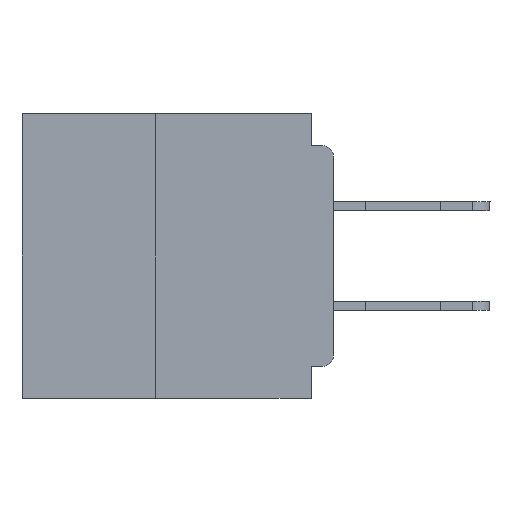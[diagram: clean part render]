
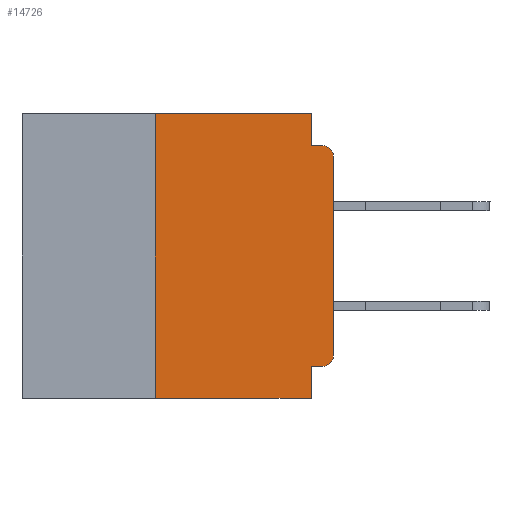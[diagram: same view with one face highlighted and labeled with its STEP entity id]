
A CAD part, left-side view. The second image highlights one B-rep face of the part: STEP entity #14726.
In plain terms, the highlighted planar face has unit normal (-1, 0, 0).
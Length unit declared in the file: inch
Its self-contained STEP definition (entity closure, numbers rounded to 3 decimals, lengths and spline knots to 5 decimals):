
#247 = VECTOR ( 'NONE', #10083, 39.37008 ) ;
#314 = FACE_OUTER_BOUND ( 'NONE', #32976, .T. ) ;
#708 = LINE ( 'NONE', #953, #49015 ) ;
#953 = CARTESIAN_POINT ( 'NONE',  ( 0., 0., -0.045 ) ) ;
#1011 = CARTESIAN_POINT ( 'NONE',  ( 0., 0.031, -0.4 ) ) ;
#1020 = LINE ( 'NONE', #16061, #47851 ) ;
#1048 = ORIENTED_EDGE ( 'NONE', *, *, #45016, .F. ) ;
#1842 = CARTESIAN_POINT ( 'NONE',  ( 0., 0.25, -0.4 ) ) ;
#2087 = DIRECTION ( 'NONE',  ( 0., 0., -1. ) ) ;
#2810 = VERTEX_POINT ( 'NONE', #1842 ) ;
#2949 = CARTESIAN_POINT ( 'NONE',  ( 0., 0.031, 0. ) ) ;
#3975 = ORIENTED_EDGE ( 'NONE', *, *, #46911, .T. ) ;
#4010 = LINE ( 'NONE', #34703, #13553 ) ;
#5346 = PLANE ( 'NONE',  #19706 ) ;
#6728 = DIRECTION ( 'NONE',  ( 0., 0., 1. ) ) ;
#7217 = CARTESIAN_POINT ( 'NONE',  ( 0., 0.031, -0.045 ) ) ;
#7301 = VERTEX_POINT ( 'NONE', #14299 ) ;
#7501 = VECTOR ( 'NONE', #6728, 39.37008 ) ;
#8438 = CARTESIAN_POINT ( 'NONE',  ( 0., 0.437, 0. ) ) ;
#10048 = DIRECTION ( 'NONE',  ( 1., 0., 0. ) ) ;
#10083 = DIRECTION ( 'NONE',  ( 0., 0., 1. ) ) ;
#10195 = VECTOR ( 'NONE', #36454, 39.37008 ) ;
#10543 = ORIENTED_EDGE ( 'NONE', *, *, #55514, .T. ) ;
#10912 = ORIENTED_EDGE ( 'NONE', *, *, #20775, .F. ) ;
#10965 = EDGE_CURVE ( 'NONE', #47925, #43229, #708, .T. ) ;
#11674 = LINE ( 'NONE', #8438, #10195 ) ;
#13553 = VECTOR ( 'NONE', #30035, 39.37008 ) ;
#14299 = CARTESIAN_POINT ( 'NONE',  ( 0., 0.015, -0.355 ) ) ;
#14620 = CARTESIAN_POINT ( 'NONE',  ( 0., 0.25, -0.4 ) ) ;
#14726 = ADVANCED_FACE ( 'NONE', ( #314 ), #5346, .F. ) ;
#14771 = DIRECTION ( 'NONE',  ( -1., 0., 0. ) ) ;
#15822 = VERTEX_POINT ( 'NONE', #45118 ) ;
#16061 = CARTESIAN_POINT ( 'NONE',  ( 0., 0., -0.355 ) ) ;
#17132 = LINE ( 'NONE', #49896, #20036 ) ;
#17173 = ORIENTED_EDGE ( 'NONE', *, *, #10965, .F. ) ;
#17838 = CARTESIAN_POINT ( 'NONE',  ( 0., 0.25, 0. ) ) ;
#19706 = AXIS2_PLACEMENT_3D ( 'NONE', #33350, #10048, #42744 ) ;
#20036 = VECTOR ( 'NONE', #21883, 39.37008 ) ;
#20775 = EDGE_CURVE ( 'NONE', #41397, #40643, #11674, .T. ) ;
#21014 = VERTEX_POINT ( 'NONE', #1011 ) ;
#21883 = DIRECTION ( 'NONE',  ( 0., 0., -1. ) ) ;
#23010 = VECTOR ( 'NONE', #2087, 39.37008 ) ;
#23017 = CARTESIAN_POINT ( 'NONE',  ( 0., 0.015, -0.06 ) ) ;
#24742 = CARTESIAN_POINT ( 'NONE',  ( 0., 0.015, -0.045 ) ) ;
#24991 = ORIENTED_EDGE ( 'NONE', *, *, #59913, .F. ) ;
#25428 = CARTESIAN_POINT ( 'NONE',  ( 0., 0.031, -0.4 ) ) ;
#27711 = DIRECTION ( 'NONE',  ( 0., 0., -1. ) ) ;
#28760 = EDGE_CURVE ( 'NONE', #2810, #41397, #36116, .T. ) ;
#28992 = DIRECTION ( 'NONE',  ( 0., -1., 0. ) ) ;
#30035 = DIRECTION ( 'NONE',  ( 0., -1., 0. ) ) ;
#31281 = CARTESIAN_POINT ( 'NONE',  ( 0., 0.031, -0.355 ) ) ;
#31881 = ORIENTED_EDGE ( 'NONE', *, *, #58664, .T. ) ;
#32976 = EDGE_LOOP ( 'NONE', ( #3975, #31881, #17173, #1048, #10912, #53333, #10543, #58263, #24991, #42939 ) ) ;
#33350 = CARTESIAN_POINT ( 'NONE',  ( 0., 0.437, 0. ) ) ;
#34703 = CARTESIAN_POINT ( 'NONE',  ( 0., 0.437, -0.4 ) ) ;
#36116 = LINE ( 'NONE', #14620, #247 ) ;
#36454 = DIRECTION ( 'NONE',  ( 0., -1., 0. ) ) ;
#36752 = AXIS2_PLACEMENT_3D ( 'NONE', #23017, #55696, #27711 ) ;
#36918 = LINE ( 'NONE', #25428, #23010 ) ;
#38842 = LINE ( 'NONE', #39471, #7501 ) ;
#39026 = CARTESIAN_POINT ( 'NONE',  ( 0., 0., -0.06 ) ) ;
#39471 = CARTESIAN_POINT ( 'NONE',  ( 0., 0., 0. ) ) ;
#40643 = VERTEX_POINT ( 'NONE', #2949 ) ;
#41397 = VERTEX_POINT ( 'NONE', #17838 ) ;
#42731 = CARTESIAN_POINT ( 'NONE',  ( 0., 0.015, -0.34 ) ) ;
#42744 = DIRECTION ( 'NONE',  ( 0., 0., -1. ) ) ;
#42939 = ORIENTED_EDGE ( 'NONE', *, *, #60372, .T. ) ;
#43229 = VERTEX_POINT ( 'NONE', #24742 ) ;
#45016 = EDGE_CURVE ( 'NONE', #40643, #47925, #17132, .T. ) ;
#45118 = CARTESIAN_POINT ( 'NONE',  ( 0., 0., -0.34 ) ) ;
#46911 = EDGE_CURVE ( 'NONE', #15822, #58309, #38842, .T. ) ;
#47440 = DIRECTION ( 'NONE',  ( 0., 0., -1. ) ) ;
#47794 = CIRCLE ( 'NONE', #48504, 0.015 ) ;
#47851 = VECTOR ( 'NONE', #53426, 39.37008 ) ;
#47925 = VERTEX_POINT ( 'NONE', #7217 ) ;
#48504 = AXIS2_PLACEMENT_3D ( 'NONE', #42731, #14771, #47440 ) ;
#48675 = VERTEX_POINT ( 'NONE', #31281 ) ;
#49015 = VECTOR ( 'NONE', #28992, 39.37008 ) ;
#49896 = CARTESIAN_POINT ( 'NONE',  ( 0., 0.031, 0. ) ) ;
#53333 = ORIENTED_EDGE ( 'NONE', *, *, #28760, .F. ) ;
#53426 = DIRECTION ( 'NONE',  ( 0., 1., 0. ) ) ;
#55514 = EDGE_CURVE ( 'NONE', #2810, #21014, #4010, .T. ) ;
#55696 = DIRECTION ( 'NONE',  ( -1., 0., 0. ) ) ;
#57487 = CIRCLE ( 'NONE', #36752, 0.015 ) ;
#58263 = ORIENTED_EDGE ( 'NONE', *, *, #59924, .F. ) ;
#58309 = VERTEX_POINT ( 'NONE', #39026 ) ;
#58664 = EDGE_CURVE ( 'NONE', #58309, #43229, #57487, .T. ) ;
#59913 = EDGE_CURVE ( 'NONE', #7301, #48675, #1020, .T. ) ;
#59924 = EDGE_CURVE ( 'NONE', #48675, #21014, #36918, .T. ) ;
#60372 = EDGE_CURVE ( 'NONE', #7301, #15822, #47794, .T. ) ;
